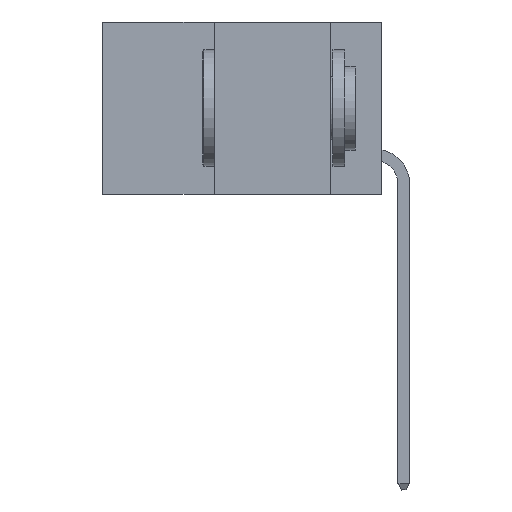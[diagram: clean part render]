
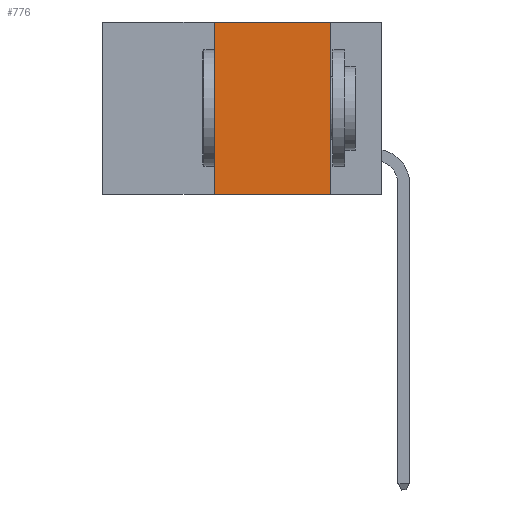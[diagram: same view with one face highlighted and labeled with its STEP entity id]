
A CAD part, left-side view. The second image highlights one B-rep face of the part: STEP entity #776.
In plain terms, the highlighted planar face has unit normal (-1, 0, 0).
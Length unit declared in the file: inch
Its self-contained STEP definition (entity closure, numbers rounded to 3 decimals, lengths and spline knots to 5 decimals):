
#776 = ADVANCED_FACE ( 'NONE', ( #13712 ), #6013, .F. ) ;
#979 = CARTESIAN_POINT ( 'NONE',  ( 0., 0.6, -0.37 ) ) ;
#998 = DIRECTION ( 'NONE',  ( 0., 0., -1. ) ) ;
#1452 = LINE ( 'NONE', #13512, #1600 ) ;
#1600 = VECTOR ( 'NONE', #12492, 39.37008 ) ;
#1983 = CARTESIAN_POINT ( 'NONE',  ( 0., 0.36, -0.37 ) ) ;
#3069 = ORIENTED_EDGE ( 'NONE', *, *, #9849, .F. ) ;
#3163 = VERTEX_POINT ( 'NONE', #1983 ) ;
#3537 = EDGE_CURVE ( 'NONE', #10214, #10152, #13453, .T. ) ;
#3661 = VERTEX_POINT ( 'NONE', #8328 ) ;
#3670 = ORIENTED_EDGE ( 'NONE', *, *, #13833, .T. ) ;
#4785 = VECTOR ( 'NONE', #6386, 39.37008 ) ;
#5451 = LINE ( 'NONE', #979, #4785 ) ;
#6013 = PLANE ( 'NONE',  #13122 ) ;
#6386 = DIRECTION ( 'NONE',  ( 0., -1., 0. ) ) ;
#6859 = VECTOR ( 'NONE', #11318, 39.37008 ) ;
#7666 = CARTESIAN_POINT ( 'NONE',  ( 0., 0.11, 0. ) ) ;
#8328 = CARTESIAN_POINT ( 'NONE',  ( 0., 0.11, -0.37 ) ) ;
#8406 = ORIENTED_EDGE ( 'NONE', *, *, #3537, .F. ) ;
#9122 = CARTESIAN_POINT ( 'NONE',  ( 0., 0.6, 0. ) ) ;
#9358 = ORIENTED_EDGE ( 'NONE', *, *, #10388, .F. ) ;
#9849 = EDGE_CURVE ( 'NONE', #3163, #10214, #1452, .T. ) ;
#10073 = CARTESIAN_POINT ( 'NONE',  ( 0., 0.36, 0. ) ) ;
#10152 = VERTEX_POINT ( 'NONE', #7666 ) ;
#10178 = DIRECTION ( 'NONE',  ( 1., 0., 0. ) ) ;
#10214 = VERTEX_POINT ( 'NONE', #10073 ) ;
#10388 = EDGE_CURVE ( 'NONE', #10152, #3661, #10718, .T. ) ;
#10433 = EDGE_LOOP ( 'NONE', ( #9358, #8406, #3069, #3670 ) ) ;
#10564 = CARTESIAN_POINT ( 'NONE',  ( 0., 0.11, 0. ) ) ;
#10718 = LINE ( 'NONE', #10564, #13259 ) ;
#11318 = DIRECTION ( 'NONE',  ( 0., -1., 0. ) ) ;
#11370 = DIRECTION ( 'NONE',  ( 0., 0., -1. ) ) ;
#12492 = DIRECTION ( 'NONE',  ( 0., 0., 1. ) ) ;
#13122 = AXIS2_PLACEMENT_3D ( 'NONE', #13482, #10178, #11370 ) ;
#13259 = VECTOR ( 'NONE', #998, 39.37008 ) ;
#13453 = LINE ( 'NONE', #9122, #6859 ) ;
#13482 = CARTESIAN_POINT ( 'NONE',  ( 0., 0.6, 0. ) ) ;
#13512 = CARTESIAN_POINT ( 'NONE',  ( 0., 0.36, 0. ) ) ;
#13712 = FACE_OUTER_BOUND ( 'NONE', #10433, .T. ) ;
#13833 = EDGE_CURVE ( 'NONE', #3163, #3661, #5451, .T. ) ;
